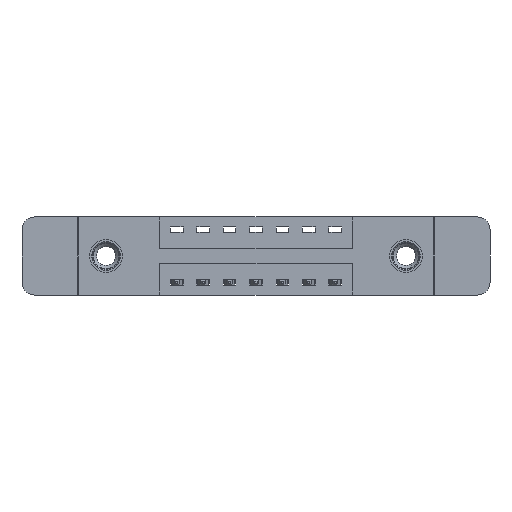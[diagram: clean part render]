
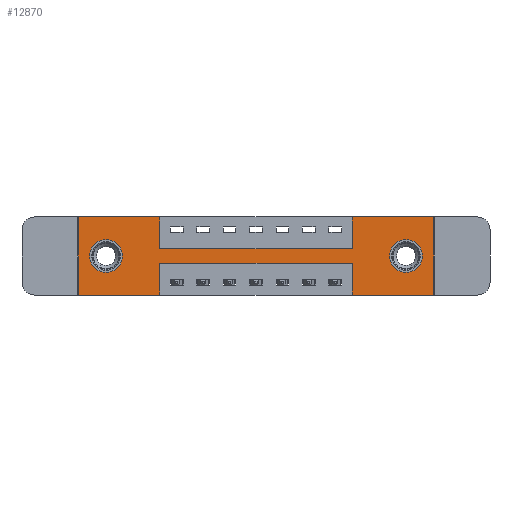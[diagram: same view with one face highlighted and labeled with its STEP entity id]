
A CAD part, front view. The second image highlights one B-rep face of the part: STEP entity #12870.
In plain terms, the highlighted planar face has unit normal (0, -1, 0).
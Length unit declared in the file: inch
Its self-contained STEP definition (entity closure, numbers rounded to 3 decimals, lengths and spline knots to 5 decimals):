
#256 = VERTEX_POINT ( 'NONE', #6283 ) ;
#267 = CARTESIAN_POINT ( 'NONE',  ( 0., 0., -0.37 ) ) ;
#339 = CARTESIAN_POINT ( 'NONE',  ( 1.2975, 0., 0. ) ) ;
#355 = CARTESIAN_POINT ( 'NONE',  ( 1.2975, 0., -0.15 ) ) ;
#398 = CARTESIAN_POINT ( 'NONE',  ( 0.1325, 0., -0.107 ) ) ;
#485 = ORIENTED_EDGE ( 'NONE', *, *, #9878, .F. ) ;
#544 = CARTESIAN_POINT ( 'NONE',  ( 0., 0., 0. ) ) ;
#548 = DIRECTION ( 'NONE',  ( 0., 0., 1. ) ) ;
#602 = LINE ( 'NONE', #8286, #9899 ) ;
#620 = ORIENTED_EDGE ( 'NONE', *, *, #14646, .T. ) ;
#661 = CIRCLE ( 'NONE', #2568, 0.078 ) ;
#790 = CARTESIAN_POINT ( 'NONE',  ( 0.3875, 0., 0. ) ) ;
#819 = LINE ( 'NONE', #12181, #5351 ) ;
#825 = ORIENTED_EDGE ( 'NONE', *, *, #2501, .F. ) ;
#1033 = AXIS2_PLACEMENT_3D ( 'NONE', #5055, #4029, #548 ) ;
#1149 = CARTESIAN_POINT ( 'NONE',  ( 1.685, 0., 0. ) ) ;
#1228 = FACE_BOUND ( 'NONE', #12279, .T. ) ;
#1342 = VERTEX_POINT ( 'NONE', #12611 ) ;
#1384 = PLANE ( 'NONE',  #4613 ) ;
#1452 = DIRECTION ( 'NONE',  ( 0., 0., -1. ) ) ;
#1531 = LINE ( 'NONE', #2899, #9753 ) ;
#1768 = CARTESIAN_POINT ( 'NONE',  ( 0., 0., -0.37 ) ) ;
#1873 = ORIENTED_EDGE ( 'NONE', *, *, #6448, .T. ) ;
#2164 = DIRECTION ( 'NONE',  ( 0., 0., 1. ) ) ;
#2185 = DIRECTION ( 'NONE',  ( 0., 0., 1. ) ) ;
#2250 = EDGE_CURVE ( 'NONE', #10376, #5655, #10853, .T. ) ;
#2285 = LINE ( 'NONE', #10352, #2779 ) ;
#2337 = VECTOR ( 'NONE', #9951, 39.37008 ) ;
#2353 = VECTOR ( 'NONE', #12048, 39.37008 ) ;
#2389 = CARTESIAN_POINT ( 'NONE',  ( 0., 0., 0. ) ) ;
#2501 = EDGE_CURVE ( 'NONE', #6420, #12785, #2285, .T. ) ;
#2568 = AXIS2_PLACEMENT_3D ( 'NONE', #3714, #5863, #6896 ) ;
#2779 = VECTOR ( 'NONE', #3370, 39.37008 ) ;
#2899 = CARTESIAN_POINT ( 'NONE',  ( 1.2975, 0., -0.37 ) ) ;
#3252 = DIRECTION ( 'NONE',  ( 0., 1., 0. ) ) ;
#3339 = EDGE_CURVE ( 'NONE', #12004, #14160, #12965, .T. ) ;
#3370 = DIRECTION ( 'NONE',  ( -1., 0., 0. ) ) ;
#3374 = EDGE_CURVE ( 'NONE', #14432, #14288, #4847, .T. ) ;
#3492 = EDGE_LOOP ( 'NONE', ( #485, #825, #7836, #13169, #9966, #3951, #8006, #8954, #11502, #7076, #6752, #7351 ) ) ;
#3524 = LINE ( 'NONE', #12615, #3603 ) ;
#3534 = CARTESIAN_POINT ( 'NONE',  ( 1.2975, 0., -0.37 ) ) ;
#3601 = CARTESIAN_POINT ( 'NONE',  ( 1.5525, 0., -0.107 ) ) ;
#3603 = VECTOR ( 'NONE', #9013, 39.37008 ) ;
#3714 = CARTESIAN_POINT ( 'NONE',  ( 1.5525, 0., -0.185 ) ) ;
#3792 = LINE ( 'NONE', #11679, #8870 ) ;
#3951 = ORIENTED_EDGE ( 'NONE', *, *, #3374, .F. ) ;
#4029 = DIRECTION ( 'NONE',  ( 0., 1., 0. ) ) ;
#4534 = DIRECTION ( 'NONE',  ( 0., 1., 0. ) ) ;
#4613 = AXIS2_PLACEMENT_3D ( 'NONE', #267, #7058, #1452 ) ;
#4682 = FACE_BOUND ( 'NONE', #13648, .T. ) ;
#4847 = LINE ( 'NONE', #544, #13280 ) ;
#5053 = DIRECTION ( 'NONE',  ( 1., 0., 0. ) ) ;
#5055 = CARTESIAN_POINT ( 'NONE',  ( 0.1325, 0., -0.185 ) ) ;
#5275 = DIRECTION ( 'NONE',  ( 0., 0., -1. ) ) ;
#5351 = VECTOR ( 'NONE', #2164, 39.37008 ) ;
#5655 = VERTEX_POINT ( 'NONE', #3601 ) ;
#5671 = CARTESIAN_POINT ( 'NONE',  ( 1.5525, 0., -0.263 ) ) ;
#5863 = DIRECTION ( 'NONE',  ( 0., 1., 0. ) ) ;
#5950 = VERTEX_POINT ( 'NONE', #790 ) ;
#6283 = CARTESIAN_POINT ( 'NONE',  ( 1.685, 0., -0.37 ) ) ;
#6351 = DIRECTION ( 'NONE',  ( 0., 0., -1. ) ) ;
#6420 = VERTEX_POINT ( 'NONE', #10873 ) ;
#6448 = EDGE_CURVE ( 'NONE', #9781, #1342, #14360, .T. ) ;
#6752 = ORIENTED_EDGE ( 'NONE', *, *, #12656, .F. ) ;
#6825 = CARTESIAN_POINT ( 'NONE',  ( 0.1325, 0., -0.185 ) ) ;
#6896 = DIRECTION ( 'NONE',  ( 0., 0., -1. ) ) ;
#7058 = DIRECTION ( 'NONE',  ( 0., -1., 0. ) ) ;
#7076 = ORIENTED_EDGE ( 'NONE', *, *, #8804, .F. ) ;
#7200 = CARTESIAN_POINT ( 'NONE',  ( 0.3875, 0., -0.22 ) ) ;
#7351 = ORIENTED_EDGE ( 'NONE', *, *, #3339, .F. ) ;
#7431 = CARTESIAN_POINT ( 'NONE',  ( 1.685, 0., 0. ) ) ;
#7476 = CARTESIAN_POINT ( 'NONE',  ( 0., 0., -0.37 ) ) ;
#7582 = EDGE_CURVE ( 'NONE', #12446, #14432, #3792, .T. ) ;
#7836 = ORIENTED_EDGE ( 'NONE', *, *, #8039, .F. ) ;
#7859 = AXIS2_PLACEMENT_3D ( 'NONE', #6825, #4534, #2185 ) ;
#8006 = ORIENTED_EDGE ( 'NONE', *, *, #7582, .F. ) ;
#8039 = EDGE_CURVE ( 'NONE', #13829, #6420, #1531, .T. ) ;
#8286 = CARTESIAN_POINT ( 'NONE',  ( 0.3875, 0., -0.37 ) ) ;
#8344 = DIRECTION ( 'NONE',  ( 0., 0., 1. ) ) ;
#8359 = ORIENTED_EDGE ( 'NONE', *, *, #10048, .T. ) ;
#8442 = VERTEX_POINT ( 'NONE', #8588 ) ;
#8588 = CARTESIAN_POINT ( 'NONE',  ( 0.3875, 0., -0.15 ) ) ;
#8589 = VERTEX_POINT ( 'NONE', #2389 ) ;
#8804 = EDGE_CURVE ( 'NONE', #8589, #5950, #13268, .T. ) ;
#8870 = VECTOR ( 'NONE', #8344, 39.37008 ) ;
#8954 = ORIENTED_EDGE ( 'NONE', *, *, #14627, .F. ) ;
#9013 = DIRECTION ( 'NONE',  ( 1., 0., 0. ) ) ;
#9207 = FACE_OUTER_BOUND ( 'NONE', #3492, .T. ) ;
#9305 = DIRECTION ( 'NONE',  ( -1., 0., 0. ) ) ;
#9523 = CARTESIAN_POINT ( 'NONE',  ( 0., 0., -0.37 ) ) ;
#9753 = VECTOR ( 'NONE', #11970, 39.37008 ) ;
#9781 = VERTEX_POINT ( 'NONE', #398 ) ;
#9871 = LINE ( 'NONE', #7476, #2353 ) ;
#9878 = EDGE_CURVE ( 'NONE', #12785, #12004, #602, .T. ) ;
#9899 = VECTOR ( 'NONE', #5275, 39.37008 ) ;
#9908 = AXIS2_PLACEMENT_3D ( 'NONE', #13457, #3252, #11060 ) ;
#9951 = DIRECTION ( 'NONE',  ( 1., 0., 0. ) ) ;
#9966 = ORIENTED_EDGE ( 'NONE', *, *, #10013, .F. ) ;
#10013 = EDGE_CURVE ( 'NONE', #14288, #256, #14626, .T. ) ;
#10048 = EDGE_CURVE ( 'NONE', #5655, #10376, #661, .T. ) ;
#10352 = CARTESIAN_POINT ( 'NONE',  ( 0.3875, 0., -0.22 ) ) ;
#10376 = VERTEX_POINT ( 'NONE', #5671 ) ;
#10441 = LINE ( 'NONE', #11992, #13102 ) ;
#10842 = EDGE_CURVE ( 'NONE', #256, #13829, #9871, .T. ) ;
#10853 = CIRCLE ( 'NONE', #9908, 0.078 ) ;
#10873 = CARTESIAN_POINT ( 'NONE',  ( 1.2975, 0., -0.22 ) ) ;
#10957 = CIRCLE ( 'NONE', #7859, 0.078 ) ;
#11060 = DIRECTION ( 'NONE',  ( 0., 0., -1. ) ) ;
#11350 = VECTOR ( 'NONE', #14409, 39.37008 ) ;
#11502 = ORIENTED_EDGE ( 'NONE', *, *, #14268, .F. ) ;
#11679 = CARTESIAN_POINT ( 'NONE',  ( 1.2975, 0., 0. ) ) ;
#11970 = DIRECTION ( 'NONE',  ( 0., 0., 1. ) ) ;
#11992 = CARTESIAN_POINT ( 'NONE',  ( 0.3875, 0., 0. ) ) ;
#12004 = VERTEX_POINT ( 'NONE', #13812 ) ;
#12048 = DIRECTION ( 'NONE',  ( -1., 0., 0. ) ) ;
#12181 = CARTESIAN_POINT ( 'NONE',  ( 0., 0., 0. ) ) ;
#12279 = EDGE_LOOP ( 'NONE', ( #8359, #12828 ) ) ;
#12446 = VERTEX_POINT ( 'NONE', #355 ) ;
#12611 = CARTESIAN_POINT ( 'NONE',  ( 0.1325, 0., -0.263 ) ) ;
#12615 = CARTESIAN_POINT ( 'NONE',  ( 0.3875, 0., -0.15 ) ) ;
#12656 = EDGE_CURVE ( 'NONE', #14160, #8589, #819, .T. ) ;
#12785 = VERTEX_POINT ( 'NONE', #7200 ) ;
#12828 = ORIENTED_EDGE ( 'NONE', *, *, #2250, .T. ) ;
#12870 = ADVANCED_FACE ( 'NONE', ( #1228, #4682, #9207 ), #1384, .T. ) ;
#12965 = LINE ( 'NONE', #9523, #14001 ) ;
#13102 = VECTOR ( 'NONE', #6351, 39.37008 ) ;
#13169 = ORIENTED_EDGE ( 'NONE', *, *, #10842, .F. ) ;
#13268 = LINE ( 'NONE', #13404, #2337 ) ;
#13280 = VECTOR ( 'NONE', #5053, 39.37008 ) ;
#13404 = CARTESIAN_POINT ( 'NONE',  ( 0., 0., 0. ) ) ;
#13457 = CARTESIAN_POINT ( 'NONE',  ( 1.5525, 0., -0.185 ) ) ;
#13648 = EDGE_LOOP ( 'NONE', ( #1873, #620 ) ) ;
#13812 = CARTESIAN_POINT ( 'NONE',  ( 0.3875, 0., -0.37 ) ) ;
#13829 = VERTEX_POINT ( 'NONE', #3534 ) ;
#14001 = VECTOR ( 'NONE', #9305, 39.37008 ) ;
#14160 = VERTEX_POINT ( 'NONE', #1768 ) ;
#14268 = EDGE_CURVE ( 'NONE', #5950, #8442, #10441, .T. ) ;
#14288 = VERTEX_POINT ( 'NONE', #7431 ) ;
#14360 = CIRCLE ( 'NONE', #1033, 0.078 ) ;
#14409 = DIRECTION ( 'NONE',  ( 0., 0., -1. ) ) ;
#14432 = VERTEX_POINT ( 'NONE', #339 ) ;
#14626 = LINE ( 'NONE', #1149, #11350 ) ;
#14627 = EDGE_CURVE ( 'NONE', #8442, #12446, #3524, .T. ) ;
#14646 = EDGE_CURVE ( 'NONE', #1342, #9781, #10957, .T. ) ;
